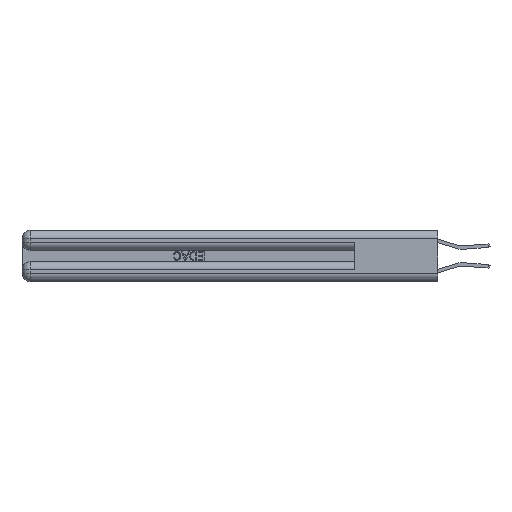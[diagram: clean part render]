
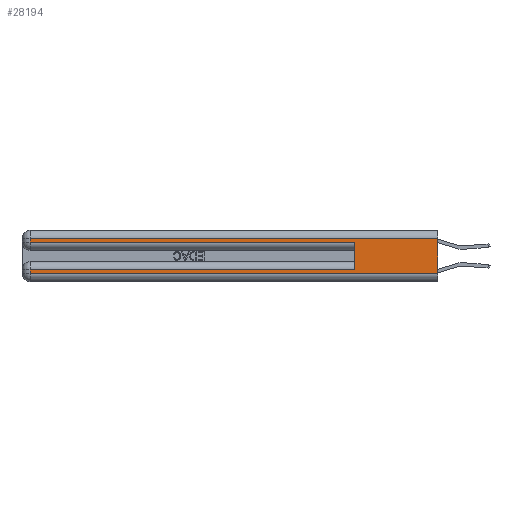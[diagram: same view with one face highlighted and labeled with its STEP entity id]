
A CAD part, left-side view. The second image highlights one B-rep face of the part: STEP entity #28194.
In plain terms, the highlighted planar face has unit normal (-1, 0, 0).
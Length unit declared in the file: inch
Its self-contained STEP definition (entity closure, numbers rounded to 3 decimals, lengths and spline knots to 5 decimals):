
#64 = AXIS2_PLACEMENT_3D ( 'NONE', #9122, #4185, #10819 ) ;
#90 = EDGE_CURVE ( 'NONE', #14287, #18930, #10698, .T. ) ;
#494 = CARTESIAN_POINT ( 'NONE',  ( 0., 2.94, 0.31 ) ) ;
#1700 = LINE ( 'NONE', #27521, #13057 ) ;
#3119 = CARTESIAN_POINT ( 'NONE',  ( 0., 2.94, 0.285 ) ) ;
#4183 = EDGE_CURVE ( 'NONE', #18807, #18930, #13496, .T. ) ;
#4185 = DIRECTION ( 'NONE',  ( 1., 0., 0. ) ) ;
#4653 = EDGE_CURVE ( 'NONE', #5457, #14287, #1700, .T. ) ;
#4878 = LINE ( 'NONE', #28959, #26756 ) ;
#5457 = VERTEX_POINT ( 'NONE', #8827 ) ;
#5913 = CARTESIAN_POINT ( 'NONE',  ( 0., 0., 0.085 ) ) ;
#6194 = PLANE ( 'NONE',  #64 ) ;
#6336 = LINE ( 'NONE', #6488, #9215 ) ;
#6433 = CARTESIAN_POINT ( 'NONE',  ( 0., 2.94, 0.06 ) ) ;
#6472 = VERTEX_POINT ( 'NONE', #494 ) ;
#6488 = CARTESIAN_POINT ( 'NONE',  ( 0., 0., 0.285 ) ) ;
#6625 = CARTESIAN_POINT ( 'NONE',  ( 0., 0.6, 0.145 ) ) ;
#7224 = EDGE_CURVE ( 'NONE', #11410, #22891, #6336, .T. ) ;
#7981 = LINE ( 'NONE', #17728, #22617 ) ;
#8827 = CARTESIAN_POINT ( 'NONE',  ( 0., 2.94, 0.085 ) ) ;
#9122 = CARTESIAN_POINT ( 'NONE',  ( 0., 0., 0.37 ) ) ;
#9215 = VECTOR ( 'NONE', #16075, 39.37008 ) ;
#10698 = LINE ( 'NONE', #20155, #24811 ) ;
#10819 = DIRECTION ( 'NONE',  ( 0., 0., -1. ) ) ;
#10894 = ORIENTED_EDGE ( 'NONE', *, *, #28836, .T. ) ;
#10947 = DIRECTION ( 'NONE',  ( 0., 0., 1. ) ) ;
#10984 = EDGE_CURVE ( 'NONE', #18807, #6472, #7981, .T. ) ;
#11019 = CARTESIAN_POINT ( 'NONE',  ( 0., 0., 0.31 ) ) ;
#11057 = VECTOR ( 'NONE', #30182, 39.37008 ) ;
#11317 = CARTESIAN_POINT ( 'NONE',  ( 0., 0., 0.06 ) ) ;
#11410 = VERTEX_POINT ( 'NONE', #3119 ) ;
#11818 = DIRECTION ( 'NONE',  ( 0., 0., -1. ) ) ;
#12250 = ORIENTED_EDGE ( 'NONE', *, *, #10984, .T. ) ;
#12284 = ORIENTED_EDGE ( 'NONE', *, *, #7224, .T. ) ;
#13057 = VECTOR ( 'NONE', #13770, 39.37008 ) ;
#13303 = LINE ( 'NONE', #5913, #28012 ) ;
#13496 = LINE ( 'NONE', #16289, #11057 ) ;
#13770 = DIRECTION ( 'NONE',  ( 0., 0., -1. ) ) ;
#13969 = EDGE_CURVE ( 'NONE', #24160, #22891, #27797, .T. ) ;
#14287 = VERTEX_POINT ( 'NONE', #6433 ) ;
#14309 = ORIENTED_EDGE ( 'NONE', *, *, #4183, .F. ) ;
#14846 = ORIENTED_EDGE ( 'NONE', *, *, #4653, .T. ) ;
#15101 = DIRECTION ( 'NONE',  ( 0., 1., 0. ) ) ;
#16075 = DIRECTION ( 'NONE',  ( 0., -1., 0. ) ) ;
#16289 = CARTESIAN_POINT ( 'NONE',  ( 0., 0., 0.37 ) ) ;
#16448 = EDGE_LOOP ( 'NONE', ( #14309, #12250, #10894, #12284, #17827, #23710, #14846, #19430 ) ) ;
#17728 = CARTESIAN_POINT ( 'NONE',  ( 0., 0., 0.31 ) ) ;
#17827 = ORIENTED_EDGE ( 'NONE', *, *, #13969, .F. ) ;
#17960 = FACE_OUTER_BOUND ( 'NONE', #16448, .T. ) ;
#18807 = VERTEX_POINT ( 'NONE', #11019 ) ;
#18930 = VERTEX_POINT ( 'NONE', #11317 ) ;
#19308 = EDGE_CURVE ( 'NONE', #24160, #5457, #13303, .T. ) ;
#19430 = ORIENTED_EDGE ( 'NONE', *, *, #90, .T. ) ;
#20155 = CARTESIAN_POINT ( 'NONE',  ( 0., 0., 0.06 ) ) ;
#21276 = VECTOR ( 'NONE', #10947, 39.37008 ) ;
#21860 = CARTESIAN_POINT ( 'NONE',  ( 0., 0.6, 0.085 ) ) ;
#21968 = CARTESIAN_POINT ( 'NONE',  ( 0., 0.6, 0.285 ) ) ;
#22617 = VECTOR ( 'NONE', #15101, 39.37008 ) ;
#22891 = VERTEX_POINT ( 'NONE', #21968 ) ;
#23710 = ORIENTED_EDGE ( 'NONE', *, *, #19308, .T. ) ;
#24160 = VERTEX_POINT ( 'NONE', #21860 ) ;
#24612 = DIRECTION ( 'NONE',  ( 0., 1., 0. ) ) ;
#24811 = VECTOR ( 'NONE', #27091, 39.37008 ) ;
#26756 = VECTOR ( 'NONE', #11818, 39.37008 ) ;
#27091 = DIRECTION ( 'NONE',  ( 0., -1., 0. ) ) ;
#27521 = CARTESIAN_POINT ( 'NONE',  ( 0., 2.94, 0.37 ) ) ;
#27797 = LINE ( 'NONE', #6625, #21276 ) ;
#28012 = VECTOR ( 'NONE', #24612, 39.37008 ) ;
#28194 = ADVANCED_FACE ( 'NONE', ( #17960 ), #6194, .F. ) ;
#28836 = EDGE_CURVE ( 'NONE', #6472, #11410, #4878, .T. ) ;
#28959 = CARTESIAN_POINT ( 'NONE',  ( 0., 2.94, 0.37 ) ) ;
#30182 = DIRECTION ( 'NONE',  ( 0., 0., -1. ) ) ;
